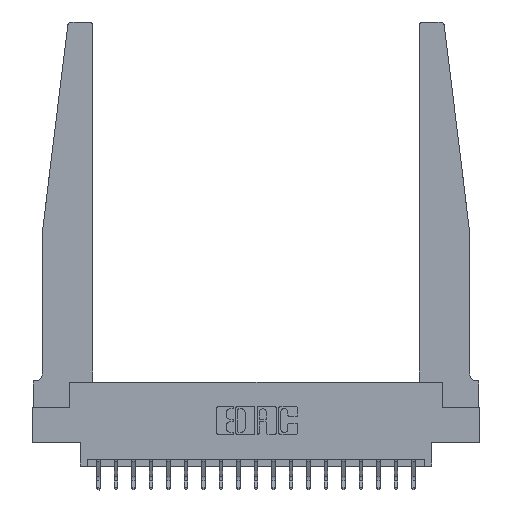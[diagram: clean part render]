
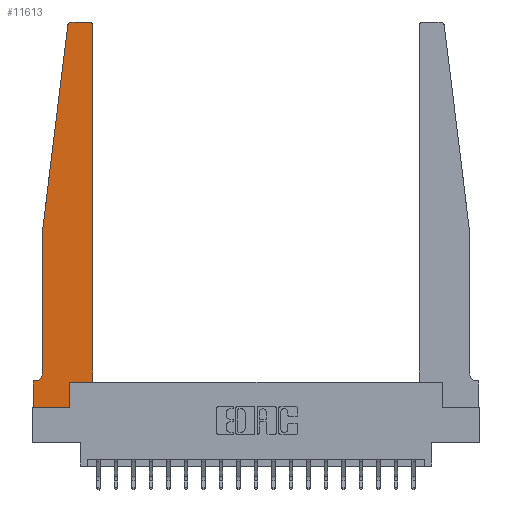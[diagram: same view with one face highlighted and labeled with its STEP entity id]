
A CAD part, top view. The second image highlights one B-rep face of the part: STEP entity #11613.
In plain terms, the highlighted planar face has unit normal (0, 0, 1).
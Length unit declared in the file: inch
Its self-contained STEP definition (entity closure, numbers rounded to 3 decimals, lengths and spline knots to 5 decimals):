
#156 = EDGE_CURVE ( 'NONE', #4785, #17580, #8167, .T. ) ;
#170 = CARTESIAN_POINT ( 'NONE',  ( 0., 0., 0.37 ) ) ;
#230 = ORIENTED_EDGE ( 'NONE', *, *, #8773, .T. ) ;
#289 = EDGE_LOOP ( 'NONE', ( #20224, #4040, #14936, #10607, #3424, #5862, #230, #3262, #3644, #4062, #20163, #14893 ) ) ;
#669 = PLANE ( 'NONE',  #2356 ) ;
#770 = CIRCLE ( 'NONE', #1257, 0.03 ) ;
#829 = CARTESIAN_POINT ( 'NONE',  ( 0.065, 1.25, 0.37 ) ) ;
#993 = CARTESIAN_POINT ( 'NONE',  ( 0.395, 2.72, 0.37 ) ) ;
#1257 = AXIS2_PLACEMENT_3D ( 'NONE', #993, #12125, #2585 ) ;
#1405 = LINE ( 'NONE', #3367, #13592 ) ;
#1491 = DIRECTION ( 'NONE',  ( 0., 1., 0. ) ) ;
#1693 = DIRECTION ( 'NONE',  ( -0.122, -0.992, 0. ) ) ;
#1760 = DIRECTION ( 'NONE',  ( -1., 0., 0. ) ) ;
#2091 = CARTESIAN_POINT ( 'NONE',  ( 0.015, 0.2375, 0.37 ) ) ;
#2356 = AXIS2_PLACEMENT_3D ( 'NONE', #16495, #14982, #5499 ) ;
#2387 = VERTEX_POINT ( 'NONE', #11137 ) ;
#2585 = DIRECTION ( 'NONE',  ( 1., 0., 0. ) ) ;
#3168 = CIRCLE ( 'NONE', #14868, 0.05 ) ;
#3262 = ORIENTED_EDGE ( 'NONE', *, *, #156, .T. ) ;
#3336 = DIRECTION ( 'NONE',  ( 0., 0., 1. ) ) ;
#3367 = CARTESIAN_POINT ( 'NONE',  ( 0.425, 0.18, 0.37 ) ) ;
#3424 = ORIENTED_EDGE ( 'NONE', *, *, #11231, .T. ) ;
#3468 = VECTOR ( 'NONE', #12901, 39.37008 ) ;
#3644 = ORIENTED_EDGE ( 'NONE', *, *, #17725, .T. ) ;
#3667 = VERTEX_POINT ( 'NONE', #12035 ) ;
#3700 = DIRECTION ( 'NONE',  ( -1., 0., 0. ) ) ;
#3715 = CARTESIAN_POINT ( 'NONE',  ( 0.27653, 2.75, 0.37 ) ) ;
#3859 = LINE ( 'NONE', #18947, #8133 ) ;
#3893 = VECTOR ( 'NONE', #7241, 39.37008 ) ;
#4040 = ORIENTED_EDGE ( 'NONE', *, *, #5374, .T. ) ;
#4059 = DIRECTION ( 'NONE',  ( 0., -1., 0. ) ) ;
#4062 = ORIENTED_EDGE ( 'NONE', *, *, #12081, .T. ) ;
#4384 = VERTEX_POINT ( 'NONE', #7267 ) ;
#4623 = CARTESIAN_POINT ( 'NONE',  ( 0.25, 2.75, 0.37 ) ) ;
#4785 = VERTEX_POINT ( 'NONE', #17739 ) ;
#5216 = VERTEX_POINT ( 'NONE', #18850 ) ;
#5359 = CARTESIAN_POINT ( 'NONE',  ( 0.2605, 0.18, 0.37 ) ) ;
#5374 = EDGE_CURVE ( 'NONE', #6895, #5216, #20274, .T. ) ;
#5400 = AXIS2_PLACEMENT_3D ( 'NONE', #12858, #3336, #14445 ) ;
#5499 = DIRECTION ( 'NONE',  ( 1., 0., 0. ) ) ;
#5787 = VECTOR ( 'NONE', #1760, 39.37008 ) ;
#5862 = ORIENTED_EDGE ( 'NONE', *, *, #19485, .T. ) ;
#6895 = VERTEX_POINT ( 'NONE', #3715 ) ;
#7009 = EDGE_CURVE ( 'NONE', #3667, #16849, #770, .T. ) ;
#7241 = DIRECTION ( 'NONE',  ( 1., 0., 0. ) ) ;
#7267 = CARTESIAN_POINT ( 'NONE',  ( 0.065, 1.25, 0.37 ) ) ;
#7269 = LINE ( 'NONE', #170, #3468 ) ;
#7522 = CARTESIAN_POINT ( 'NONE',  ( 0., 0., 0.37 ) ) ;
#7554 = CARTESIAN_POINT ( 'NONE',  ( 0.2605, 0., 0.37 ) ) ;
#7636 = EDGE_CURVE ( 'NONE', #4384, #16573, #9966, .T. ) ;
#8133 = VECTOR ( 'NONE', #1491, 39.37008 ) ;
#8167 = LINE ( 'NONE', #7522, #3893 ) ;
#8297 = EDGE_CURVE ( 'NONE', #2387, #3667, #14880, .T. ) ;
#8482 = EDGE_CURVE ( 'NONE', #5216, #4384, #19663, .T. ) ;
#8773 = EDGE_CURVE ( 'NONE', #15690, #4785, #7269, .T. ) ;
#8888 = VECTOR ( 'NONE', #17294, 39.37008 ) ;
#9490 = VECTOR ( 'NONE', #4059, 39.37008 ) ;
#9662 = CARTESIAN_POINT ( 'NONE',  ( 0.065, 1.25, 0.37 ) ) ;
#9966 = LINE ( 'NONE', #829, #9490 ) ;
#10607 = ORIENTED_EDGE ( 'NONE', *, *, #7636, .T. ) ;
#10902 = CARTESIAN_POINT ( 'NONE',  ( 0.015, 0.1875, 0.37 ) ) ;
#11137 = CARTESIAN_POINT ( 'NONE',  ( 0.425, 0.18, 0.37 ) ) ;
#11231 = EDGE_CURVE ( 'NONE', #16573, #11917, #3168, .T. ) ;
#11305 = CARTESIAN_POINT ( 'NONE',  ( 0.065, 0.1875, 0.37 ) ) ;
#11308 = DIRECTION ( 'NONE',  ( 1., 0., 0. ) ) ;
#11613 = ADVANCED_FACE ( 'NONE', ( #13106 ), #669, .T. ) ;
#11917 = VERTEX_POINT ( 'NONE', #10902 ) ;
#12035 = CARTESIAN_POINT ( 'NONE',  ( 0.425, 2.72, 0.37 ) ) ;
#12081 = EDGE_CURVE ( 'NONE', #15158, #2387, #1405, .T. ) ;
#12125 = DIRECTION ( 'NONE',  ( 0., 0., 1. ) ) ;
#12213 = DIRECTION ( 'NONE',  ( 0., 1., 0. ) ) ;
#12553 = LINE ( 'NONE', #4623, #8888 ) ;
#12858 = CARTESIAN_POINT ( 'NONE',  ( 0.27653, 2.72, 0.37 ) ) ;
#12901 = DIRECTION ( 'NONE',  ( 0., -1., 0. ) ) ;
#13098 = EDGE_CURVE ( 'NONE', #16849, #6895, #12553, .T. ) ;
#13106 = FACE_OUTER_BOUND ( 'NONE', #289, .T. ) ;
#13217 = DIRECTION ( 'NONE',  ( 0., 0., -1. ) ) ;
#13592 = VECTOR ( 'NONE', #11308, 39.37008 ) ;
#13681 = CARTESIAN_POINT ( 'NONE',  ( 0.065, 0.2375, 0.37 ) ) ;
#13745 = CARTESIAN_POINT ( 'NONE',  ( 0.425, 0.18, 0.37 ) ) ;
#14382 = VECTOR ( 'NONE', #12213, 39.37008 ) ;
#14445 = DIRECTION ( 'NONE',  ( 1., 0., 0. ) ) ;
#14561 = CARTESIAN_POINT ( 'NONE',  ( 0.395, 2.75, 0.37 ) ) ;
#14868 = AXIS2_PLACEMENT_3D ( 'NONE', #2091, #13217, #3700 ) ;
#14880 = LINE ( 'NONE', #13745, #14382 ) ;
#14893 = ORIENTED_EDGE ( 'NONE', *, *, #7009, .T. ) ;
#14936 = ORIENTED_EDGE ( 'NONE', *, *, #8482, .T. ) ;
#14982 = DIRECTION ( 'NONE',  ( 0., 0., 1. ) ) ;
#15158 = VERTEX_POINT ( 'NONE', #5359 ) ;
#15402 = VECTOR ( 'NONE', #1693, 39.37008 ) ;
#15690 = VERTEX_POINT ( 'NONE', #16190 ) ;
#16190 = CARTESIAN_POINT ( 'NONE',  ( 0., 0.1875, 0.37 ) ) ;
#16495 = CARTESIAN_POINT ( 'NONE',  ( 0., 0.1875, 0.37 ) ) ;
#16573 = VERTEX_POINT ( 'NONE', #13681 ) ;
#16849 = VERTEX_POINT ( 'NONE', #14561 ) ;
#17294 = DIRECTION ( 'NONE',  ( -1., 0., 0. ) ) ;
#17580 = VERTEX_POINT ( 'NONE', #7554 ) ;
#17725 = EDGE_CURVE ( 'NONE', #17580, #15158, #3859, .T. ) ;
#17739 = CARTESIAN_POINT ( 'NONE',  ( 0., 0., 0.37 ) ) ;
#17928 = LINE ( 'NONE', #11305, #5787 ) ;
#18850 = CARTESIAN_POINT ( 'NONE',  ( 0.24675, 2.72367, 0.37 ) ) ;
#18947 = CARTESIAN_POINT ( 'NONE',  ( 0.2605, 0.18, 0.37 ) ) ;
#19485 = EDGE_CURVE ( 'NONE', #11917, #15690, #17928, .T. ) ;
#19663 = LINE ( 'NONE', #9662, #15402 ) ;
#20163 = ORIENTED_EDGE ( 'NONE', *, *, #8297, .T. ) ;
#20224 = ORIENTED_EDGE ( 'NONE', *, *, #13098, .T. ) ;
#20274 = CIRCLE ( 'NONE', #5400, 0.03 ) ;
